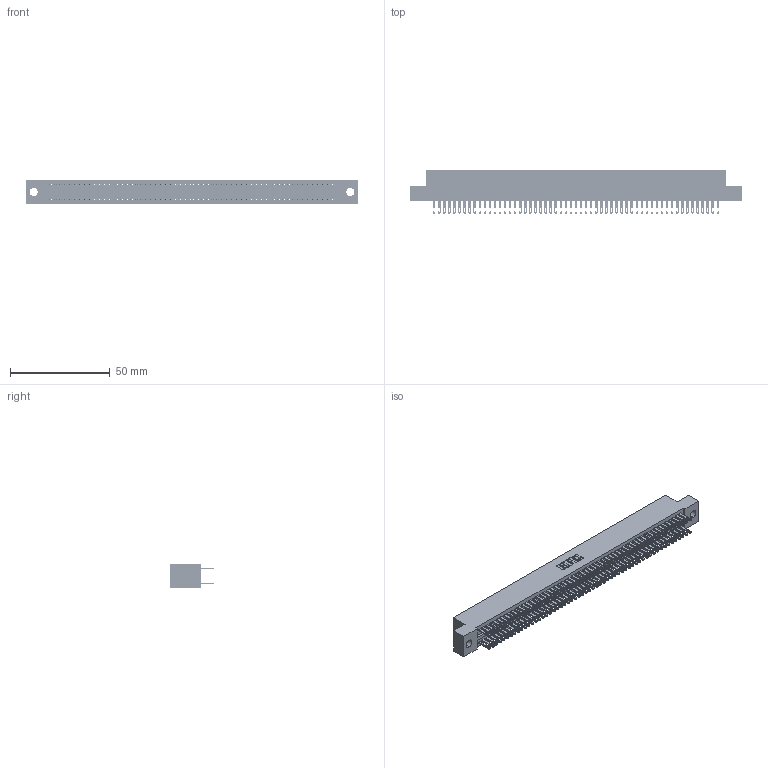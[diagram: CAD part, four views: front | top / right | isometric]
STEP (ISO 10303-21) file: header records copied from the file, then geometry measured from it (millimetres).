
FILE_DESCRIPTION (( 'STEP AP203' ), '1' );
FILE_NAME ('325-114-500-209.STEP', '2020-02-25T08:02:32', ( '' ), ( '' ), 'SwSTEP 2.0', 'SolidWorks 2016', '' );
FILE_SCHEMA (( 'CONFIG_CONTROL_DESIGN' ));
Length unit declared in the file: inch
Products named in the file (3): 325-114-500-209; 325 Part_.160 TH; 325-292-001_325-293-100
Assembly tree (115 placements, depth 2):
  325-114-500-209
    325 Part_.160 TH
    325-292-001_325-293-100  x114
Bounding box: 166.5 x 21.84 x 12.45 mm (x, y, z)
Volume: 21746.2 mm3; surface area: 27789 mm2
Topology: 115 solids, 115 shells, 5586 faces, 17069 edges, 11378 vertices
Faces by surface type: plane 3490, cylinder 2096
Entity records: 34663 total; most frequent: CARTESIAN_POINT 5726, ORIENTED_EDGE 5662, DIRECTION 4867, EDGE_CURVE 2831, LINE 2699, VECTOR 2699, VERTEX_POINT 1886, AXIS2_PLACEMENT_3D 1084
